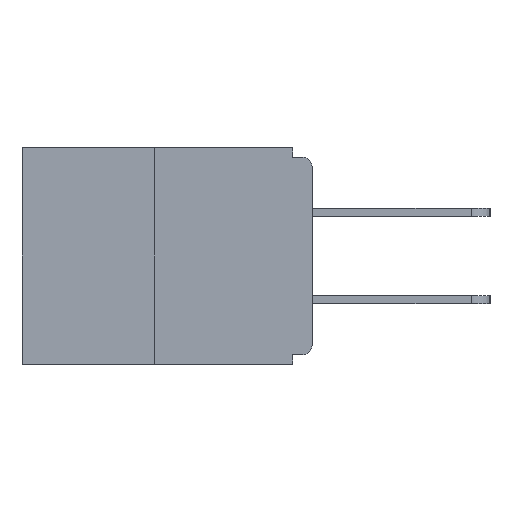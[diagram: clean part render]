
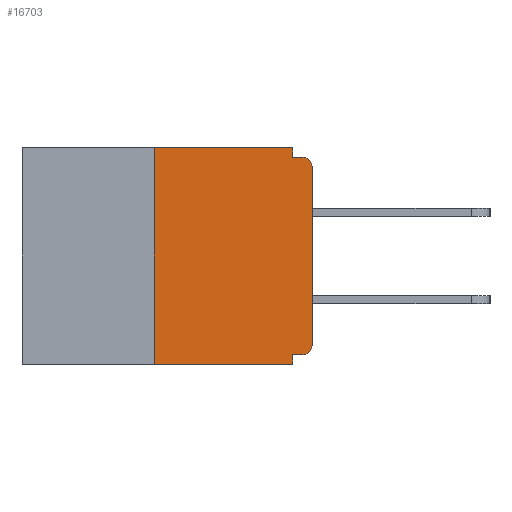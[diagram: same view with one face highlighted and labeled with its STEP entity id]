
A CAD part, left-side view. The second image highlights one B-rep face of the part: STEP entity #16703.
In plain terms, the highlighted planar face has unit normal (-1, 0, 0).
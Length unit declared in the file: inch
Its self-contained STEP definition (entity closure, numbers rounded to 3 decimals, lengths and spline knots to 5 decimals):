
#235 = DIRECTION ( 'NONE',  ( 0., -1., 0. ) ) ;
#399 = CARTESIAN_POINT ( 'NONE',  ( 0., 0.015, -0.313 ) ) ;
#1543 = EDGE_LOOP ( 'NONE', ( #5120, #12804, #1844, #14383, #8011, #21785, #7005, #18925, #4455, #19930 ) ) ;
#1844 = ORIENTED_EDGE ( 'NONE', *, *, #12287, .T. ) ;
#2097 = VERTEX_POINT ( 'NONE', #20153 ) ;
#2126 = VERTEX_POINT ( 'NONE', #16698 ) ;
#2266 = EDGE_CURVE ( 'NONE', #21989, #14260, #5295, .T. ) ;
#3141 = CARTESIAN_POINT ( 'NONE',  ( 0., 0., 0. ) ) ;
#3670 = CARTESIAN_POINT ( 'NONE',  ( 0., 0.015, -0.328 ) ) ;
#3843 = DIRECTION ( 'NONE',  ( -1., 0., 0. ) ) ;
#4005 = EDGE_CURVE ( 'NONE', #24305, #2097, #4299, .T. ) ;
#4299 = CIRCLE ( 'NONE', #23959, 0.015 ) ;
#4455 = ORIENTED_EDGE ( 'NONE', *, *, #13199, .F. ) ;
#4715 = LINE ( 'NONE', #13651, #21756 ) ;
#5120 = ORIENTED_EDGE ( 'NONE', *, *, #17423, .F. ) ;
#5140 = LINE ( 'NONE', #23204, #20391 ) ;
#5295 = CIRCLE ( 'NONE', #6624, 0.015 ) ;
#6297 = CARTESIAN_POINT ( 'NONE',  ( 0., 0.031, 0. ) ) ;
#6624 = AXIS2_PLACEMENT_3D ( 'NONE', #17347, #19137, #17258 ) ;
#7005 = ORIENTED_EDGE ( 'NONE', *, *, #10443, .T. ) ;
#7211 = VERTEX_POINT ( 'NONE', #12331 ) ;
#7275 = VECTOR ( 'NONE', #23297, 39.37008 ) ;
#7323 = VECTOR ( 'NONE', #17193, 39.37008 ) ;
#7353 = DIRECTION ( 'NONE',  ( 0., 0., -1. ) ) ;
#8011 = ORIENTED_EDGE ( 'NONE', *, *, #14978, .F. ) ;
#8506 = CARTESIAN_POINT ( 'NONE',  ( 0., 0.031, -0.343 ) ) ;
#9071 = DIRECTION ( 'NONE',  ( 0., 0., -1. ) ) ;
#9644 = VECTOR ( 'NONE', #9071, 39.37008 ) ;
#10443 = EDGE_CURVE ( 'NONE', #2097, #21989, #22657, .T. ) ;
#10560 = CARTESIAN_POINT ( 'NONE',  ( 0., 0.031, -0.015 ) ) ;
#10573 = LINE ( 'NONE', #11616, #7323 ) ;
#11286 = CARTESIAN_POINT ( 'NONE',  ( 0., 0.031, 0. ) ) ;
#11461 = CARTESIAN_POINT ( 'NONE',  ( 0., 0.015, -0.015 ) ) ;
#11616 = CARTESIAN_POINT ( 'NONE',  ( 0., 0.46, -0.343 ) ) ;
#11796 = EDGE_CURVE ( 'NONE', #20035, #21013, #14637, .T. ) ;
#12287 = EDGE_CURVE ( 'NONE', #2126, #7211, #10573, .T. ) ;
#12331 = CARTESIAN_POINT ( 'NONE',  ( 0., 0.031, -0.343 ) ) ;
#12804 = ORIENTED_EDGE ( 'NONE', *, *, #23070, .F. ) ;
#13199 = EDGE_CURVE ( 'NONE', #21013, #14260, #19618, .T. ) ;
#13445 = LINE ( 'NONE', #8506, #9644 ) ;
#13651 = CARTESIAN_POINT ( 'NONE',  ( 0., 0.46, 0. ) ) ;
#13707 = AXIS2_PLACEMENT_3D ( 'NONE', #14981, #14828, #7353 ) ;
#14260 = VERTEX_POINT ( 'NONE', #11461 ) ;
#14383 = ORIENTED_EDGE ( 'NONE', *, *, #21084, .F. ) ;
#14637 = LINE ( 'NONE', #6297, #7275 ) ;
#14687 = VERTEX_POINT ( 'NONE', #17328 ) ;
#14828 = DIRECTION ( 'NONE',  ( 1., 0., 0. ) ) ;
#14978 = EDGE_CURVE ( 'NONE', #24305, #14687, #18940, .T. ) ;
#14981 = CARTESIAN_POINT ( 'NONE',  ( 0., 0.46, 0. ) ) ;
#15109 = VECTOR ( 'NONE', #24078, 39.37008 ) ;
#15169 = DIRECTION ( 'NONE',  ( 0., -1., 0. ) ) ;
#16698 = CARTESIAN_POINT ( 'NONE',  ( 0., 0.25, -0.343 ) ) ;
#16703 = ADVANCED_FACE ( 'NONE', ( #23848 ), #22137, .F. ) ;
#17053 = CARTESIAN_POINT ( 'NONE',  ( 0., 0.25, 0. ) ) ;
#17193 = DIRECTION ( 'NONE',  ( 0., -1., 0. ) ) ;
#17253 = DIRECTION ( 'NONE',  ( 0., 0., -1. ) ) ;
#17258 = DIRECTION ( 'NONE',  ( 0., 0., -1. ) ) ;
#17328 = CARTESIAN_POINT ( 'NONE',  ( 0., 0.031, -0.328 ) ) ;
#17347 = CARTESIAN_POINT ( 'NONE',  ( 0., 0.015, -0.03 ) ) ;
#17423 = EDGE_CURVE ( 'NONE', #20689, #20035, #4715, .T. ) ;
#18094 = DIRECTION ( 'NONE',  ( 0., 0., 1. ) ) ;
#18861 = CARTESIAN_POINT ( 'NONE',  ( 0., 0., -0.015 ) ) ;
#18925 = ORIENTED_EDGE ( 'NONE', *, *, #2266, .T. ) ;
#18940 = LINE ( 'NONE', #22349, #15109 ) ;
#19137 = DIRECTION ( 'NONE',  ( -1., 0., 0. ) ) ;
#19618 = LINE ( 'NONE', #18861, #24030 ) ;
#19930 = ORIENTED_EDGE ( 'NONE', *, *, #11796, .F. ) ;
#20026 = CARTESIAN_POINT ( 'NONE',  ( 0., 0., -0.03 ) ) ;
#20035 = VERTEX_POINT ( 'NONE', #11286 ) ;
#20153 = CARTESIAN_POINT ( 'NONE',  ( 0., 0., -0.313 ) ) ;
#20391 = VECTOR ( 'NONE', #22778, 39.37008 ) ;
#20689 = VERTEX_POINT ( 'NONE', #17053 ) ;
#21013 = VERTEX_POINT ( 'NONE', #10560 ) ;
#21084 = EDGE_CURVE ( 'NONE', #14687, #7211, #13445, .T. ) ;
#21489 = VECTOR ( 'NONE', #18094, 39.37008 ) ;
#21756 = VECTOR ( 'NONE', #235, 39.37008 ) ;
#21785 = ORIENTED_EDGE ( 'NONE', *, *, #4005, .T. ) ;
#21989 = VERTEX_POINT ( 'NONE', #20026 ) ;
#22137 = PLANE ( 'NONE',  #13707 ) ;
#22349 = CARTESIAN_POINT ( 'NONE',  ( 0., 0., -0.328 ) ) ;
#22657 = LINE ( 'NONE', #3141, #21489 ) ;
#22778 = DIRECTION ( 'NONE',  ( 0., 0., 1. ) ) ;
#23070 = EDGE_CURVE ( 'NONE', #2126, #20689, #5140, .T. ) ;
#23204 = CARTESIAN_POINT ( 'NONE',  ( 0., 0.25, 0. ) ) ;
#23297 = DIRECTION ( 'NONE',  ( 0., 0., -1. ) ) ;
#23848 = FACE_OUTER_BOUND ( 'NONE', #1543, .T. ) ;
#23959 = AXIS2_PLACEMENT_3D ( 'NONE', #399, #3843, #17253 ) ;
#24030 = VECTOR ( 'NONE', #15169, 39.37008 ) ;
#24078 = DIRECTION ( 'NONE',  ( 0., 1., 0. ) ) ;
#24305 = VERTEX_POINT ( 'NONE', #3670 ) ;
